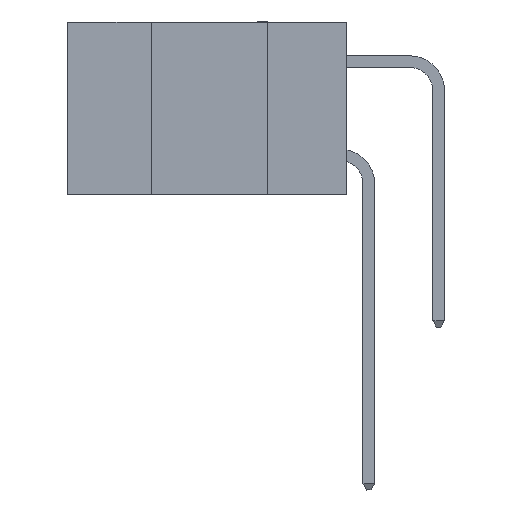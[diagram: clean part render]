
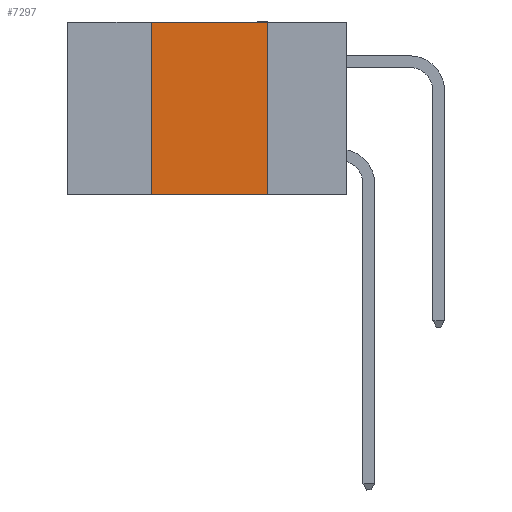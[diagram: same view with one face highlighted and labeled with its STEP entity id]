
A CAD part, left-side view. The second image highlights one B-rep face of the part: STEP entity #7297.
In plain terms, the highlighted planar face has unit normal (-1, 0, 0).
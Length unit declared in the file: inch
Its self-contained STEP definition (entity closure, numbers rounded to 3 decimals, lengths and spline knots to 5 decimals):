
#159 = EDGE_LOOP ( 'NONE', ( #5002, #11350, #4709, #11591 ) ) ;
#207 = VERTEX_POINT ( 'NONE', #31783 ) ;
#619 = PLANE ( 'NONE',  #5032 ) ;
#1086 = VERTEX_POINT ( 'NONE', #1356 ) ;
#1356 = CARTESIAN_POINT ( 'NONE',  ( 0., 0.42, 0. ) ) ;
#2291 = VECTOR ( 'NONE', #9693, 39.37008 ) ;
#3135 = FACE_OUTER_BOUND ( 'NONE', #159, .T. ) ;
#3299 = DIRECTION ( 'NONE',  ( 0., -1., 0. ) ) ;
#4709 = ORIENTED_EDGE ( 'NONE', *, *, #11761, .F. ) ;
#5002 = ORIENTED_EDGE ( 'NONE', *, *, #12145, .F. ) ;
#5032 = AXIS2_PLACEMENT_3D ( 'NONE', #25875, #13069, #26199 ) ;
#6062 = CARTESIAN_POINT ( 'NONE',  ( 0., 0.6, 0. ) ) ;
#6507 = CARTESIAN_POINT ( 'NONE',  ( 0., 0.17, 0. ) ) ;
#7211 = EDGE_CURVE ( 'NONE', #207, #29689, #8200, .T. ) ;
#7297 = ADVANCED_FACE ( 'NONE', ( #3135 ), #619, .F. ) ;
#8200 = LINE ( 'NONE', #16088, #29688 ) ;
#9693 = DIRECTION ( 'NONE',  ( 0., 0., -1. ) ) ;
#11272 = DIRECTION ( 'NONE',  ( 0., -1., 0. ) ) ;
#11350 = ORIENTED_EDGE ( 'NONE', *, *, #22750, .F. ) ;
#11591 = ORIENTED_EDGE ( 'NONE', *, *, #7211, .T. ) ;
#11761 = EDGE_CURVE ( 'NONE', #207, #1086, #32611, .T. ) ;
#12145 = EDGE_CURVE ( 'NONE', #25664, #29689, #14892, .T. ) ;
#13069 = DIRECTION ( 'NONE',  ( 1., 0., 0. ) ) ;
#14892 = LINE ( 'NONE', #32737, #2291 ) ;
#16088 = CARTESIAN_POINT ( 'NONE',  ( 0., 0.6, -0.37 ) ) ;
#18108 = CARTESIAN_POINT ( 'NONE',  ( 0., 0.17, -0.37 ) ) ;
#21371 = LINE ( 'NONE', #6062, #26353 ) ;
#22507 = CARTESIAN_POINT ( 'NONE',  ( 0., 0.42, 0. ) ) ;
#22750 = EDGE_CURVE ( 'NONE', #1086, #25664, #21371, .T. ) ;
#25664 = VERTEX_POINT ( 'NONE', #6507 ) ;
#25875 = CARTESIAN_POINT ( 'NONE',  ( 0., 0.6, 0. ) ) ;
#26199 = DIRECTION ( 'NONE',  ( 0., 0., -1. ) ) ;
#26353 = VECTOR ( 'NONE', #11272, 39.37008 ) ;
#28590 = VECTOR ( 'NONE', #30088, 39.37008 ) ;
#29688 = VECTOR ( 'NONE', #3299, 39.37008 ) ;
#29689 = VERTEX_POINT ( 'NONE', #18108 ) ;
#30088 = DIRECTION ( 'NONE',  ( 0., 0., 1. ) ) ;
#31783 = CARTESIAN_POINT ( 'NONE',  ( 0., 0.42, -0.37 ) ) ;
#32611 = LINE ( 'NONE', #22507, #28590 ) ;
#32737 = CARTESIAN_POINT ( 'NONE',  ( 0., 0.17, 0. ) ) ;
